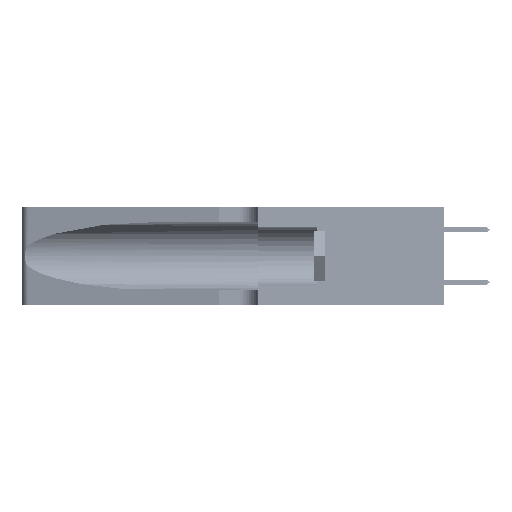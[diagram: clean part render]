
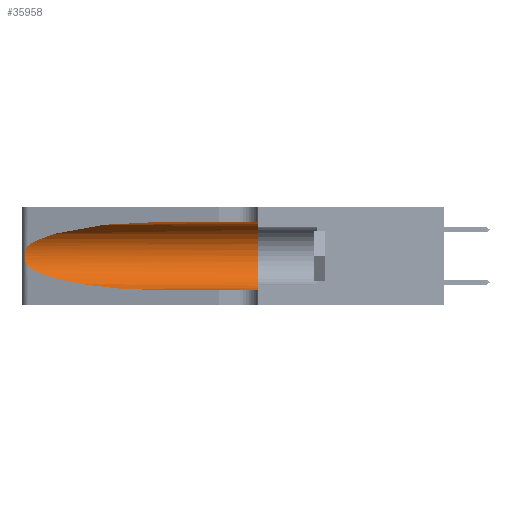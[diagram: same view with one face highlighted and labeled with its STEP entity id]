
A CAD part, left-side view. The second image highlights one B-rep face of the part: STEP entity #35958.
In plain terms, the highlighted cylindrical face has radius 3.308 mm (diameter 6.617 mm), a partial arc.
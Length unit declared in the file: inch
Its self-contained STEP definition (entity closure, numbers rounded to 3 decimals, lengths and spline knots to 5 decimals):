
#749 = DIRECTION ( 'NONE',  ( 0., -1., 0. ) ) ;
#778 = CARTESIAN_POINT ( 'NONE',  ( 0.1305, 0.72297, 0.05475 ) ) ;
#881 = EDGE_CURVE ( 'NONE', #10725, #5363, #32944, .T. ) ;
#1923 = EDGE_CURVE ( 'NONE', #16878, #16393, #52835, .T. ) ;
#2664 = ORIENTED_EDGE ( 'NONE', *, *, #39429, .F. ) ;
#2745 = CARTESIAN_POINT ( 'NONE',  ( 0.25639, 1.23186, 0.15144 ) ) ;
#5344 = EDGE_LOOP ( 'NONE', ( #20013, #8601, #31884, #25515, #25745, #2664 ) ) ;
#5363 = VERTEX_POINT ( 'NONE', #48634 ) ;
#5377 = CARTESIAN_POINT ( 'NONE',  ( 0.2373, 1.15595, 0.08982 ) ) ;
#5572 = CARTESIAN_POINT ( 'NONE',  ( 0.18966, 0.96281, 0.05475 ) ) ;
#8276 = VECTOR ( 'NONE', #47741, 39.37008 ) ;
#8601 = ORIENTED_EDGE ( 'NONE', *, *, #49157, .T. ) ;
#9256 = CARTESIAN_POINT ( 'NONE',  ( 0.25487, 1.22718, 0.22369 ) ) ;
#9536 = CARTESIAN_POINT ( 'NONE',  ( 0.1305, 0.72297, 0.05475 ) ) ;
#10725 = VERTEX_POINT ( 'NONE', #778 ) ;
#12703 = B_SPLINE_CURVE_WITH_KNOTS ( 'NONE', 3,
 ( #35410, #47852, #48021, #23607, #23061, #52530, #51997, #48202, #23419, #23246, #39907, #2745, #27958, #48555 ),
 .UNSPECIFIED., .F., .F.,
 ( 4, 2, 2, 2, 2, 2, 4 ),
 ( 0., 0.00027, 0.00053, 0.00107, 0.0016, 0.00187, 0.00214 ),
 .UNSPECIFIED. ) ;
#12980 = EDGE_CURVE ( 'NONE', #49837, #10725, #26336, .T. ) ;
#13101 = CARTESIAN_POINT ( 'NONE',  ( 0.1305, 0.72297, 0.31525 ) ) ;
#13614 = CARTESIAN_POINT ( 'NONE',  ( 0.1305, 1.61858, 0.185 ) ) ;
#14378 = CARTESIAN_POINT ( 'NONE',  ( 0.1305, 0.72297, 0.31525 ) ) ;
#14442 = VECTOR ( 'NONE', #50074, 39.37008 ) ;
#15720 = LINE ( 'NONE', #41080, #14442 ) ;
#16393 = VERTEX_POINT ( 'NONE', #33413 ) ;
#16878 = VERTEX_POINT ( 'NONE', #14378 ) ;
#17957 = CARTESIAN_POINT ( 'NONE',  ( 0.2373, 1.15595, 0.28018 ) ) ;
#17993 = CYLINDRICAL_SURFACE ( 'NONE', #50444, 0.13025 ) ;
#18604 = CARTESIAN_POINT ( 'NONE',  ( 0.1305, 1.61858, 0.05475 ) ) ;
#20013 = ORIENTED_EDGE ( 'NONE', *, *, #1923, .T. ) ;
#20656 = CARTESIAN_POINT ( 'NONE',  ( 0.1305, 0.35, 0.31525 ) ) ;
#23061 = CARTESIAN_POINT ( 'NONE',  ( 0.25854, 1.2359, 0.20912 ) ) ;
#23246 = CARTESIAN_POINT ( 'NONE',  ( 0.25856, 1.23593, 0.16098 ) ) ;
#23419 = CARTESIAN_POINT ( 'NONE',  ( 0.26017, 1.23833, 0.17102 ) ) ;
#23607 = CARTESIAN_POINT ( 'NONE',  ( 0.25787, 1.23484, 0.2124 ) ) ;
#23778 = VERTEX_POINT ( 'NONE', #20656 ) ;
#25515 = ORIENTED_EDGE ( 'NONE', *, *, #881, .T. ) ;
#25745 = ORIENTED_EDGE ( 'NONE', *, *, #26679, .F. ) ;
#26336 =( BOUNDED_CURVE ( )  B_SPLINE_CURVE ( 3, ( #42696, #5377, #5572, #9536 ),
 .UNSPECIFIED., .F., .F. ) 
 B_SPLINE_CURVE_WITH_KNOTS ( ( 4, 4 ),
 ( 3.44316, 4.71239 ),
 .UNSPECIFIED. ) 
 CURVE ( )  GEOMETRIC_REPRESENTATION_ITEM ( )  RATIONAL_B_SPLINE_CURVE ( ( 1., 0.87, 0.87, 1. ) ) 
 REPRESENTATION_ITEM ( '' )  );
#26679 = EDGE_CURVE ( 'NONE', #23778, #5363, #36470, .T. ) ;
#27518 = CARTESIAN_POINT ( 'NONE',  ( 0.1305, 0.35, 0.185 ) ) ;
#27886 = DIRECTION ( 'NONE',  ( 0., 0., 1. ) ) ;
#27958 = CARTESIAN_POINT ( 'NONE',  ( 0.25555, 1.22993, 0.14849 ) ) ;
#30287 = DIRECTION ( 'NONE',  ( 0., 0., -1. ) ) ;
#31884 = ORIENTED_EDGE ( 'NONE', *, *, #12980, .T. ) ;
#32944 = LINE ( 'NONE', #18604, #8276 ) ;
#33413 = CARTESIAN_POINT ( 'NONE',  ( 0.25487, 1.22718, 0.22369 ) ) ;
#35410 = CARTESIAN_POINT ( 'NONE',  ( 0.25487, 1.22718, 0.22369 ) ) ;
#35690 = AXIS2_PLACEMENT_3D ( 'NONE', #27518, #52634, #27886 ) ;
#35958 = ADVANCED_FACE ( 'NONE', ( #36774 ), #17993, .F. ) ;
#36470 = CIRCLE ( 'NONE', #35690, 0.13025 ) ;
#36774 = FACE_OUTER_BOUND ( 'NONE', #5344, .T. ) ;
#39429 = EDGE_CURVE ( 'NONE', #16878, #23778, #15720, .T. ) ;
#39907 = CARTESIAN_POINT ( 'NONE',  ( 0.25789, 1.23486, 0.15765 ) ) ;
#41080 = CARTESIAN_POINT ( 'NONE',  ( 0.1305, 1.61858, 0.31525 ) ) ;
#42077 = CARTESIAN_POINT ( 'NONE',  ( 0.18966, 0.96281, 0.31525 ) ) ;
#42696 = CARTESIAN_POINT ( 'NONE',  ( 0.25487, 1.22718, 0.14631 ) ) ;
#47741 = DIRECTION ( 'NONE',  ( 0., -1., 0. ) ) ;
#47852 = CARTESIAN_POINT ( 'NONE',  ( 0.25555, 1.22994, 0.2215 ) ) ;
#48021 = CARTESIAN_POINT ( 'NONE',  ( 0.25639, 1.23184, 0.21858 ) ) ;
#48202 = CARTESIAN_POINT ( 'NONE',  ( 0.26075, 1.23896, 0.178 ) ) ;
#48555 = CARTESIAN_POINT ( 'NONE',  ( 0.25487, 1.22718, 0.14631 ) ) ;
#48634 = CARTESIAN_POINT ( 'NONE',  ( 0.1305, 0.35, 0.05475 ) ) ;
#49157 = EDGE_CURVE ( 'NONE', #16393, #49837, #12703, .T. ) ;
#49837 = VERTEX_POINT ( 'NONE', #49875 ) ;
#49875 = CARTESIAN_POINT ( 'NONE',  ( 0.25487, 1.22718, 0.14631 ) ) ;
#50074 = DIRECTION ( 'NONE',  ( 0., -1., 0. ) ) ;
#50444 = AXIS2_PLACEMENT_3D ( 'NONE', #13614, #749, #30287 ) ;
#51997 = CARTESIAN_POINT ( 'NONE',  ( 0.26075, 1.23896, 0.19203 ) ) ;
#52530 = CARTESIAN_POINT ( 'NONE',  ( 0.26018, 1.23835, 0.19895 ) ) ;
#52634 = DIRECTION ( 'NONE',  ( 0., 1., 0. ) ) ;
#52835 =( BOUNDED_CURVE ( )  B_SPLINE_CURVE ( 3, ( #13101, #42077, #17957, #9256 ),
 .UNSPECIFIED., .F., .T. ) 
 B_SPLINE_CURVE_WITH_KNOTS ( ( 4, 4 ),
 ( 1.5708, 2.84003 ),
 .UNSPECIFIED. ) 
 CURVE ( )  GEOMETRIC_REPRESENTATION_ITEM ( )  RATIONAL_B_SPLINE_CURVE ( ( 1., 0.87, 0.87, 1. ) ) 
 REPRESENTATION_ITEM ( '' )  );
